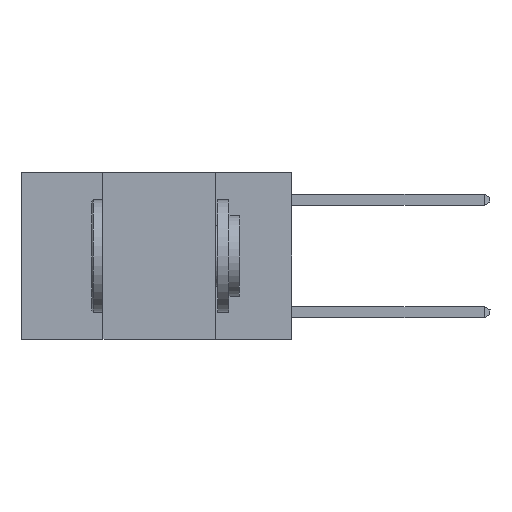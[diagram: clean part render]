
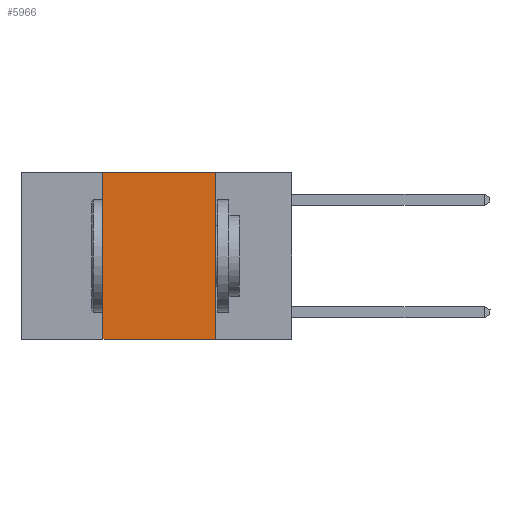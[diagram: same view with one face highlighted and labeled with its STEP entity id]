
A CAD part, left-side view. The second image highlights one B-rep face of the part: STEP entity #5966.
In plain terms, the highlighted planar face has unit normal (-1, 0, 0).
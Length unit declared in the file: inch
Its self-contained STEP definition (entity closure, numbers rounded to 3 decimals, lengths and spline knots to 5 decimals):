
#758 = AXIS2_PLACEMENT_3D ( 'NONE', #12791, #14720, #2950 ) ;
#2115 = VERTEX_POINT ( 'NONE', #12354 ) ;
#2122 = EDGE_CURVE ( 'NONE', #24375, #10750, #22449, .T. ) ;
#2527 = CARTESIAN_POINT ( 'NONE',  ( 0., 0.42, 0. ) ) ;
#2950 = DIRECTION ( 'NONE',  ( 0., 0., -1. ) ) ;
#3782 = CARTESIAN_POINT ( 'NONE',  ( 0., 0.42, 0. ) ) ;
#3813 = CARTESIAN_POINT ( 'NONE',  ( 0., 0.17, 0. ) ) ;
#4533 = DIRECTION ( 'NONE',  ( 0., 0., 1. ) ) ;
#4649 = CARTESIAN_POINT ( 'NONE',  ( 0., 0.17, 0. ) ) ;
#4887 = CARTESIAN_POINT ( 'NONE',  ( 0., 0.6, -0.37 ) ) ;
#5594 = LINE ( 'NONE', #3813, #20469 ) ;
#5966 = ADVANCED_FACE ( 'NONE', ( #22014 ), #22333, .F. ) ;
#7087 = VECTOR ( 'NONE', #4533, 39.37008 ) ;
#10091 = EDGE_CURVE ( 'NONE', #21726, #2115, #5594, .T. ) ;
#10750 = VERTEX_POINT ( 'NONE', #3782 ) ;
#11147 = ORIENTED_EDGE ( 'NONE', *, *, #10091, .F. ) ;
#11339 = ORIENTED_EDGE ( 'NONE', *, *, #17076, .F. ) ;
#11433 = ORIENTED_EDGE ( 'NONE', *, *, #2122, .F. ) ;
#11578 = VECTOR ( 'NONE', #24226, 39.37008 ) ;
#11645 = EDGE_LOOP ( 'NONE', ( #11147, #11339, #11433, #11722 ) ) ;
#11722 = ORIENTED_EDGE ( 'NONE', *, *, #18303, .T. ) ;
#12186 = LINE ( 'NONE', #4887, #11578 ) ;
#12354 = CARTESIAN_POINT ( 'NONE',  ( 0., 0.17, -0.37 ) ) ;
#12791 = CARTESIAN_POINT ( 'NONE',  ( 0., 0.6, 0. ) ) ;
#14720 = DIRECTION ( 'NONE',  ( 1., 0., 0. ) ) ;
#15850 = CARTESIAN_POINT ( 'NONE',  ( 0., 0.6, 0. ) ) ;
#17076 = EDGE_CURVE ( 'NONE', #10750, #21726, #25078, .T. ) ;
#18303 = EDGE_CURVE ( 'NONE', #24375, #2115, #12186, .T. ) ;
#18848 = VECTOR ( 'NONE', #19708, 39.37008 ) ;
#19708 = DIRECTION ( 'NONE',  ( 0., -1., 0. ) ) ;
#20144 = CARTESIAN_POINT ( 'NONE',  ( 0., 0.42, -0.37 ) ) ;
#20469 = VECTOR ( 'NONE', #21302, 39.37008 ) ;
#21302 = DIRECTION ( 'NONE',  ( 0., 0., -1. ) ) ;
#21726 = VERTEX_POINT ( 'NONE', #4649 ) ;
#22014 = FACE_OUTER_BOUND ( 'NONE', #11645, .T. ) ;
#22333 = PLANE ( 'NONE',  #758 ) ;
#22449 = LINE ( 'NONE', #2527, #7087 ) ;
#24226 = DIRECTION ( 'NONE',  ( 0., -1., 0. ) ) ;
#24375 = VERTEX_POINT ( 'NONE', #20144 ) ;
#25078 = LINE ( 'NONE', #15850, #18848 ) ;
